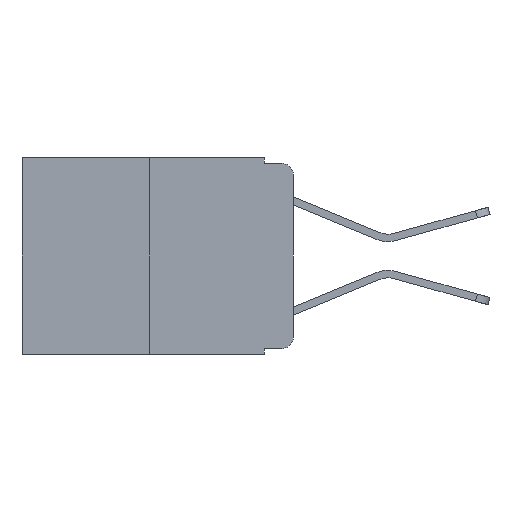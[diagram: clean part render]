
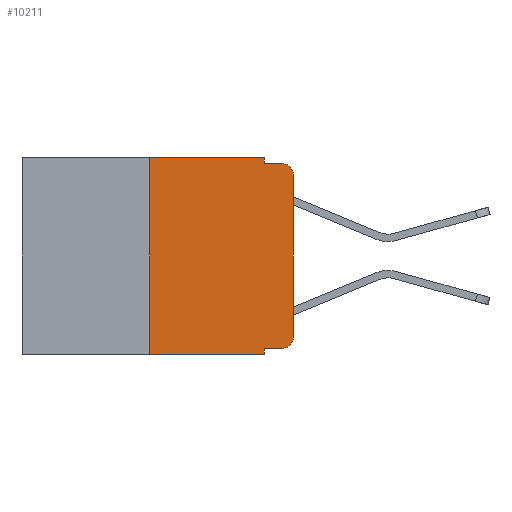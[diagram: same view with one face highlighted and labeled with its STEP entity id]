
A CAD part, left-side view. The second image highlights one B-rep face of the part: STEP entity #10211.
In plain terms, the highlighted planar face has unit normal (-1, 0, 0).
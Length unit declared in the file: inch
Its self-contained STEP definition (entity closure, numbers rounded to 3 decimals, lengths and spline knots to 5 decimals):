
#15 = CARTESIAN_POINT ( 'NONE',  ( 0., 0.02, -0.333 ) ) ;
#100 = ORIENTED_EDGE ( 'NONE', *, *, #3367, .T. ) ;
#269 = CARTESIAN_POINT ( 'NONE',  ( 0., 0.051, 0. ) ) ;
#287 = AXIS2_PLACEMENT_3D ( 'NONE', #5020, #10764, #5930 ) ;
#379 = ORIENTED_EDGE ( 'NONE', *, *, #3921, .T. ) ;
#560 = CIRCLE ( 'NONE', #4975, 0.02 ) ;
#570 = EDGE_CURVE ( 'NONE', #6763, #1109, #4592, .T. ) ;
#789 = CARTESIAN_POINT ( 'NONE',  ( 0., 0.25, 0. ) ) ;
#1046 = CARTESIAN_POINT ( 'NONE',  ( 0., 0.473, 0. ) ) ;
#1109 = VERTEX_POINT ( 'NONE', #2814 ) ;
#1209 = DIRECTION ( 'NONE',  ( 0., 0., -1. ) ) ;
#1542 = EDGE_CURVE ( 'NONE', #2599, #7312, #2554, .T. ) ;
#1549 = VERTEX_POINT ( 'NONE', #15 ) ;
#1669 = LINE ( 'NONE', #2411, #8267 ) ;
#1729 = CARTESIAN_POINT ( 'NONE',  ( 0., 0., -0.03 ) ) ;
#1945 = VECTOR ( 'NONE', #4610, 39.37008 ) ;
#2012 = VERTEX_POINT ( 'NONE', #4340 ) ;
#2141 = LINE ( 'NONE', #9005, #4166 ) ;
#2266 = VECTOR ( 'NONE', #8164, 39.37008 ) ;
#2289 = VECTOR ( 'NONE', #1209, 39.37008 ) ;
#2411 = CARTESIAN_POINT ( 'NONE',  ( 0., 0.051, -0.01 ) ) ;
#2465 = VERTEX_POINT ( 'NONE', #6381 ) ;
#2554 = LINE ( 'NONE', #3873, #2266 ) ;
#2591 = CARTESIAN_POINT ( 'NONE',  ( 0., 0.25, -0.343 ) ) ;
#2599 = VERTEX_POINT ( 'NONE', #6115 ) ;
#2633 = ORIENTED_EDGE ( 'NONE', *, *, #6161, .F. ) ;
#2814 = CARTESIAN_POINT ( 'NONE',  ( 0., 0.051, -0.01 ) ) ;
#2815 = DIRECTION ( 'NONE',  ( 1., 0., 0. ) ) ;
#3115 = EDGE_CURVE ( 'NONE', #8324, #7312, #8774, .T. ) ;
#3139 = EDGE_CURVE ( 'NONE', #1109, #2465, #1669, .T. ) ;
#3367 = EDGE_CURVE ( 'NONE', #2599, #1549, #6694, .T. ) ;
#3707 = VECTOR ( 'NONE', #6035, 39.37008 ) ;
#3873 = CARTESIAN_POINT ( 'NONE',  ( 0., 0.051, 0. ) ) ;
#3921 = EDGE_CURVE ( 'NONE', #9933, #8346, #3948, .T. ) ;
#3948 = LINE ( 'NONE', #7023, #8243 ) ;
#3975 = LINE ( 'NONE', #789, #3707 ) ;
#4057 = EDGE_LOOP ( 'NONE', ( #379, #5908, #4378, #10456, #2633, #5777, #10109, #10337, #100, #9509 ) ) ;
#4166 = VECTOR ( 'NONE', #10560, 39.37008 ) ;
#4304 = CARTESIAN_POINT ( 'NONE',  ( 0., 0.02, -0.03 ) ) ;
#4340 = CARTESIAN_POINT ( 'NONE',  ( 0., 0.25, 0. ) ) ;
#4378 = ORIENTED_EDGE ( 'NONE', *, *, #3139, .F. ) ;
#4590 = CARTESIAN_POINT ( 'NONE',  ( 0., 0.473, -0.343 ) ) ;
#4592 = LINE ( 'NONE', #269, #2289 ) ;
#4610 = DIRECTION ( 'NONE',  ( 0., -1., 0. ) ) ;
#4628 = DIRECTION ( 'NONE',  ( 0., -1., 0. ) ) ;
#4946 = FACE_OUTER_BOUND ( 'NONE', #4057, .T. ) ;
#4951 = CIRCLE ( 'NONE', #287, 0.02 ) ;
#4975 = AXIS2_PLACEMENT_3D ( 'NONE', #4304, #10127, #5185 ) ;
#5020 = CARTESIAN_POINT ( 'NONE',  ( 0., 0.02, -0.313 ) ) ;
#5185 = DIRECTION ( 'NONE',  ( 0., 0., -1. ) ) ;
#5777 = ORIENTED_EDGE ( 'NONE', *, *, #9512, .F. ) ;
#5908 = ORIENTED_EDGE ( 'NONE', *, *, #10606, .T. ) ;
#5930 = DIRECTION ( 'NONE',  ( 0., 0., -1. ) ) ;
#6035 = DIRECTION ( 'NONE',  ( 0., 0., 1. ) ) ;
#6115 = CARTESIAN_POINT ( 'NONE',  ( 0., 0.051, -0.333 ) ) ;
#6161 = EDGE_CURVE ( 'NONE', #2012, #6763, #2141, .T. ) ;
#6381 = CARTESIAN_POINT ( 'NONE',  ( 0., 0.02, -0.01 ) ) ;
#6694 = LINE ( 'NONE', #7608, #8398 ) ;
#6763 = VERTEX_POINT ( 'NONE', #10541 ) ;
#7023 = CARTESIAN_POINT ( 'NONE',  ( 0., 0., 0. ) ) ;
#7055 = DIRECTION ( 'NONE',  ( 0., 0., 1. ) ) ;
#7312 = VERTEX_POINT ( 'NONE', #9692 ) ;
#7374 = DIRECTION ( 'NONE',  ( 0., -1., 0. ) ) ;
#7608 = CARTESIAN_POINT ( 'NONE',  ( 0., 0.051, -0.333 ) ) ;
#7954 = PLANE ( 'NONE',  #8239 ) ;
#8164 = DIRECTION ( 'NONE',  ( 0., 0., -1. ) ) ;
#8175 = EDGE_CURVE ( 'NONE', #1549, #9933, #4951, .T. ) ;
#8239 = AXIS2_PLACEMENT_3D ( 'NONE', #1046, #2815, #8769 ) ;
#8243 = VECTOR ( 'NONE', #7055, 39.37008 ) ;
#8267 = VECTOR ( 'NONE', #4628, 39.37008 ) ;
#8324 = VERTEX_POINT ( 'NONE', #2591 ) ;
#8346 = VERTEX_POINT ( 'NONE', #1729 ) ;
#8398 = VECTOR ( 'NONE', #7374, 39.37008 ) ;
#8769 = DIRECTION ( 'NONE',  ( 0., 0., -1. ) ) ;
#8774 = LINE ( 'NONE', #4590, #1945 ) ;
#9005 = CARTESIAN_POINT ( 'NONE',  ( 0., 0.473, 0. ) ) ;
#9274 = CARTESIAN_POINT ( 'NONE',  ( 0., 0., -0.313 ) ) ;
#9509 = ORIENTED_EDGE ( 'NONE', *, *, #8175, .T. ) ;
#9512 = EDGE_CURVE ( 'NONE', #8324, #2012, #3975, .T. ) ;
#9692 = CARTESIAN_POINT ( 'NONE',  ( 0., 0.051, -0.343 ) ) ;
#9933 = VERTEX_POINT ( 'NONE', #9274 ) ;
#10109 = ORIENTED_EDGE ( 'NONE', *, *, #3115, .T. ) ;
#10127 = DIRECTION ( 'NONE',  ( -1., 0., 0. ) ) ;
#10211 = ADVANCED_FACE ( 'NONE', ( #4946 ), #7954, .F. ) ;
#10337 = ORIENTED_EDGE ( 'NONE', *, *, #1542, .F. ) ;
#10456 = ORIENTED_EDGE ( 'NONE', *, *, #570, .F. ) ;
#10541 = CARTESIAN_POINT ( 'NONE',  ( 0., 0.051, 0. ) ) ;
#10560 = DIRECTION ( 'NONE',  ( 0., -1., 0. ) ) ;
#10606 = EDGE_CURVE ( 'NONE', #8346, #2465, #560, .T. ) ;
#10764 = DIRECTION ( 'NONE',  ( -1., 0., 0. ) ) ;
